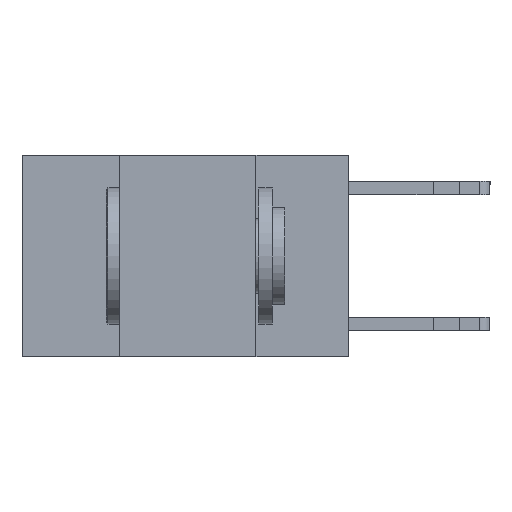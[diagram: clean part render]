
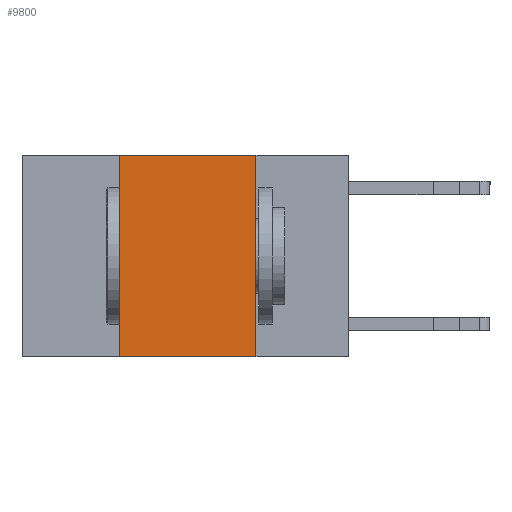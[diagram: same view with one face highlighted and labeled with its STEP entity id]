
A CAD part, left-side view. The second image highlights one B-rep face of the part: STEP entity #9800.
In plain terms, the highlighted planar face has unit normal (-1, 0, 0).
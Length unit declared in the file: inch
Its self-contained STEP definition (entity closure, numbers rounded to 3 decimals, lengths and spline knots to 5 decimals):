
#156 = AXIS2_PLACEMENT_3D ( 'NONE', #20578, #6295, #16205 ) ;
#777 = LINE ( 'NONE', #15456, #891 ) ;
#881 = CARTESIAN_POINT ( 'NONE',  ( 0., 0.42, 0. ) ) ;
#891 = VECTOR ( 'NONE', #13859, 39.37008 ) ;
#2489 = ORIENTED_EDGE ( 'NONE', *, *, #7415, .F. ) ;
#3605 = LINE ( 'NONE', #19446, #4481 ) ;
#4481 = VECTOR ( 'NONE', #14793, 39.37008 ) ;
#4538 = DIRECTION ( 'NONE',  ( 0., 0., 1. ) ) ;
#4609 = VECTOR ( 'NONE', #13660, 39.37008 ) ;
#5034 = VERTEX_POINT ( 'NONE', #8829 ) ;
#6295 = DIRECTION ( 'NONE',  ( 1., 0., 0. ) ) ;
#7415 = EDGE_CURVE ( 'NONE', #12302, #20798, #12250, .T. ) ;
#7531 = ORIENTED_EDGE ( 'NONE', *, *, #15199, .F. ) ;
#7723 = VECTOR ( 'NONE', #4538, 39.37008 ) ;
#8467 = CARTESIAN_POINT ( 'NONE',  ( 0., 0.42, -0.37 ) ) ;
#8829 = CARTESIAN_POINT ( 'NONE',  ( 0., 0.17, 0. ) ) ;
#9800 = ADVANCED_FACE ( 'NONE', ( #11157 ), #11252, .F. ) ;
#11157 = FACE_OUTER_BOUND ( 'NONE', #17381, .T. ) ;
#11252 = PLANE ( 'NONE',  #156 ) ;
#12213 = EDGE_CURVE ( 'NONE', #20798, #5034, #3605, .T. ) ;
#12250 = LINE ( 'NONE', #12347, #7723 ) ;
#12302 = VERTEX_POINT ( 'NONE', #8467 ) ;
#12347 = CARTESIAN_POINT ( 'NONE',  ( 0., 0.42, 0. ) ) ;
#13349 = CARTESIAN_POINT ( 'NONE',  ( 0., 0.6, -0.37 ) ) ;
#13660 = DIRECTION ( 'NONE',  ( 0., -1., 0. ) ) ;
#13859 = DIRECTION ( 'NONE',  ( 0., 0., -1. ) ) ;
#14244 = ORIENTED_EDGE ( 'NONE', *, *, #16995, .T. ) ;
#14793 = DIRECTION ( 'NONE',  ( 0., -1., 0. ) ) ;
#15199 = EDGE_CURVE ( 'NONE', #5034, #16567, #777, .T. ) ;
#15456 = CARTESIAN_POINT ( 'NONE',  ( 0., 0.17, 0. ) ) ;
#16205 = DIRECTION ( 'NONE',  ( 0., 0., -1. ) ) ;
#16567 = VERTEX_POINT ( 'NONE', #16862 ) ;
#16630 = LINE ( 'NONE', #13349, #4609 ) ;
#16862 = CARTESIAN_POINT ( 'NONE',  ( 0., 0.17, -0.37 ) ) ;
#16995 = EDGE_CURVE ( 'NONE', #12302, #16567, #16630, .T. ) ;
#17381 = EDGE_LOOP ( 'NONE', ( #7531, #20284, #2489, #14244 ) ) ;
#19446 = CARTESIAN_POINT ( 'NONE',  ( 0., 0.6, 0. ) ) ;
#20284 = ORIENTED_EDGE ( 'NONE', *, *, #12213, .F. ) ;
#20578 = CARTESIAN_POINT ( 'NONE',  ( 0., 0.6, 0. ) ) ;
#20798 = VERTEX_POINT ( 'NONE', #881 ) ;
